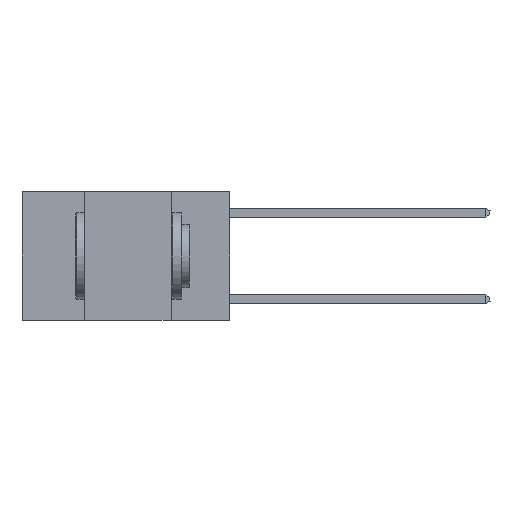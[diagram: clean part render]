
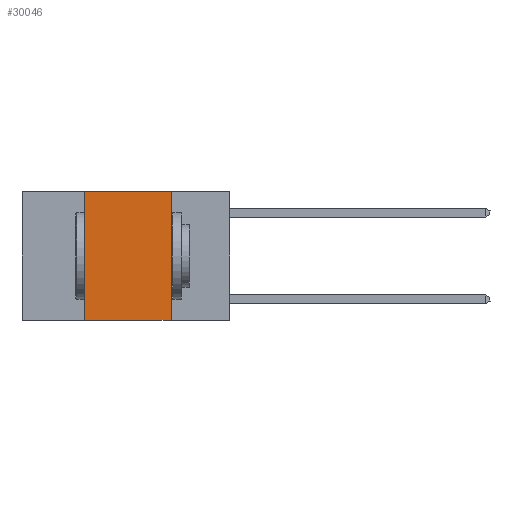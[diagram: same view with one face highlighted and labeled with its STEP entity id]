
A CAD part, left-side view. The second image highlights one B-rep face of the part: STEP entity #30046.
In plain terms, the highlighted planar face has unit normal (-1, 0, 0).
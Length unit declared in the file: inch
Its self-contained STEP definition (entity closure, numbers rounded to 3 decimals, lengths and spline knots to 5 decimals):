
#2516 = PLANE ( 'NONE',  #18332 ) ;
#2819 = VERTEX_POINT ( 'NONE', #22516 ) ;
#4057 = DIRECTION ( 'NONE',  ( 0., -1., 0. ) ) ;
#5410 = VECTOR ( 'NONE', #17726, 39.37008 ) ;
#6237 = VECTOR ( 'NONE', #13365, 39.37008 ) ;
#6994 = CARTESIAN_POINT ( 'NONE',  ( 0., 0.17, 0. ) ) ;
#9182 = CARTESIAN_POINT ( 'NONE',  ( 0., 0.17, -0.37 ) ) ;
#9186 = CARTESIAN_POINT ( 'NONE',  ( 0., 0.42, -0.37 ) ) ;
#9689 = DIRECTION ( 'NONE',  ( 0., 0., -1. ) ) ;
#10905 = LINE ( 'NONE', #20357, #5410 ) ;
#11872 = EDGE_LOOP ( 'NONE', ( #22262, #18136, #15791, #19366 ) ) ;
#12103 = EDGE_CURVE ( 'NONE', #12333, #23209, #10905, .T. ) ;
#12162 = CARTESIAN_POINT ( 'NONE',  ( 0., 0.6, 0. ) ) ;
#12262 = EDGE_CURVE ( 'NONE', #19913, #23209, #26263, .T. ) ;
#12333 = VERTEX_POINT ( 'NONE', #9186 ) ;
#13238 = VECTOR ( 'NONE', #4057, 39.37008 ) ;
#13365 = DIRECTION ( 'NONE',  ( 0., 0., 1. ) ) ;
#13658 = LINE ( 'NONE', #20617, #6237 ) ;
#15565 = CARTESIAN_POINT ( 'NONE',  ( 0., 0.17, 0. ) ) ;
#15791 = ORIENTED_EDGE ( 'NONE', *, *, #23566, .F. ) ;
#16465 = DIRECTION ( 'NONE',  ( 0., 0., -1. ) ) ;
#17726 = DIRECTION ( 'NONE',  ( 0., -1., 0. ) ) ;
#18136 = ORIENTED_EDGE ( 'NONE', *, *, #24498, .F. ) ;
#18332 = AXIS2_PLACEMENT_3D ( 'NONE', #12162, #21141, #9689 ) ;
#18480 = CARTESIAN_POINT ( 'NONE',  ( 0., 0.6, 0. ) ) ;
#18812 = FACE_OUTER_BOUND ( 'NONE', #11872, .T. ) ;
#19366 = ORIENTED_EDGE ( 'NONE', *, *, #12103, .T. ) ;
#19913 = VERTEX_POINT ( 'NONE', #15565 ) ;
#20357 = CARTESIAN_POINT ( 'NONE',  ( 0., 0.6, -0.37 ) ) ;
#20617 = CARTESIAN_POINT ( 'NONE',  ( 0., 0.42, 0. ) ) ;
#21141 = DIRECTION ( 'NONE',  ( 1., 0., 0. ) ) ;
#22262 = ORIENTED_EDGE ( 'NONE', *, *, #12262, .F. ) ;
#22516 = CARTESIAN_POINT ( 'NONE',  ( 0., 0.42, 0. ) ) ;
#23209 = VERTEX_POINT ( 'NONE', #9182 ) ;
#23566 = EDGE_CURVE ( 'NONE', #12333, #2819, #13658, .T. ) ;
#24498 = EDGE_CURVE ( 'NONE', #2819, #19913, #30047, .T. ) ;
#26263 = LINE ( 'NONE', #6994, #29286 ) ;
#29286 = VECTOR ( 'NONE', #16465, 39.37008 ) ;
#30046 = ADVANCED_FACE ( 'NONE', ( #18812 ), #2516, .F. ) ;
#30047 = LINE ( 'NONE', #18480, #13238 ) ;
